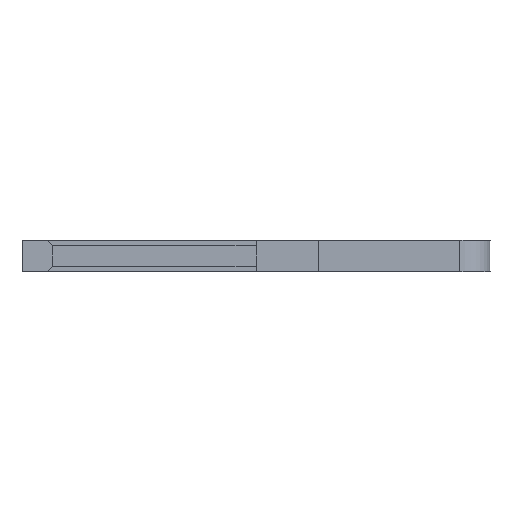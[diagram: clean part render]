
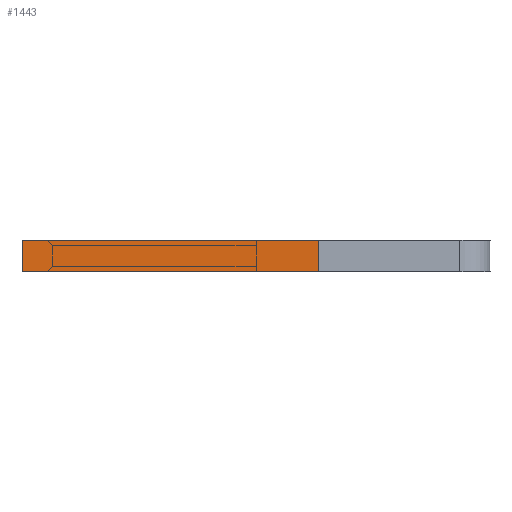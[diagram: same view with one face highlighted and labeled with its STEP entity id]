
A CAD part, left-side view. The second image highlights one B-rep face of the part: STEP entity #1443.
In plain terms, the highlighted face is planar.
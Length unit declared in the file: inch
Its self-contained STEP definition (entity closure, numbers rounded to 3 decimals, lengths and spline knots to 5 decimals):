
#244 = VERTEX_POINT ( 'NONE', #1079 ) ;
#296 = EDGE_CURVE ( 'NONE', #2512, #3378, #2258, .T. ) ;
#384 = DIRECTION ( 'NONE',  ( 0., 1., 0. ) ) ;
#651 = ORIENTED_EDGE ( 'NONE', *, *, #2189, .F. ) ;
#654 = CARTESIAN_POINT ( 'NONE',  ( -0.01, 0.15, -0.04 ) ) ;
#676 = ORIENTED_EDGE ( 'NONE', *, *, #1287, .T. ) ;
#684 = LINE ( 'NONE', #1186, #3525 ) ;
#754 = AXIS2_PLACEMENT_3D ( 'NONE', #3221, #3492, #1765 ) ;
#759 = VECTOR ( 'NONE', #2547, 39.37008 ) ;
#926 = VECTOR ( 'NONE', #384, 39.37008 ) ;
#1079 = CARTESIAN_POINT ( 'NONE',  ( 0.01, 0.15, -0.04 ) ) ;
#1186 = CARTESIAN_POINT ( 'NONE',  ( 0.01, 0.15, -0.04 ) ) ;
#1196 = DIRECTION ( 'NONE',  ( -1., 0., 0. ) ) ;
#1287 = EDGE_CURVE ( 'NONE', #3378, #2867, #2703, .T. ) ;
#1443 = ADVANCED_FACE ( 'NONE', ( #1454 ), #1450, .F. ) ;
#1450 = PLANE ( 'NONE',  #754 ) ;
#1454 = FACE_OUTER_BOUND ( 'NONE', #3390, .T. ) ;
#1765 = DIRECTION ( 'NONE',  ( 1., 0., 0. ) ) ;
#1893 = EDGE_CURVE ( 'NONE', #244, #2867, #684, .T. ) ;
#2053 = ORIENTED_EDGE ( 'NONE', *, *, #1893, .F. ) ;
#2136 = ORIENTED_EDGE ( 'NONE', *, *, #296, .T. ) ;
#2189 = EDGE_CURVE ( 'NONE', #2512, #244, #3687, .T. ) ;
#2258 = LINE ( 'NONE', #3716, #759 ) ;
#2263 = CARTESIAN_POINT ( 'NONE',  ( -0.01, 0.15, -0.04 ) ) ;
#2493 = CARTESIAN_POINT ( 'NONE',  ( -0.01, -0.04, -0.04 ) ) ;
#2512 = VERTEX_POINT ( 'NONE', #3599 ) ;
#2547 = DIRECTION ( 'NONE',  ( -1., 0., 0. ) ) ;
#2554 = DIRECTION ( 'NONE',  ( 0., 1., 0. ) ) ;
#2703 = LINE ( 'NONE', #2263, #3263 ) ;
#2867 = VERTEX_POINT ( 'NONE', #654 ) ;
#3221 = CARTESIAN_POINT ( 'NONE',  ( 0.01, 0.15, -0.04 ) ) ;
#3262 = CARTESIAN_POINT ( 'NONE',  ( 0.01, 0.15, -0.04 ) ) ;
#3263 = VECTOR ( 'NONE', #2554, 39.37008 ) ;
#3378 = VERTEX_POINT ( 'NONE', #2493 ) ;
#3390 = EDGE_LOOP ( 'NONE', ( #676, #2053, #651, #2136 ) ) ;
#3492 = DIRECTION ( 'NONE',  ( 0., 0., 1. ) ) ;
#3525 = VECTOR ( 'NONE', #1196, 39.37008 ) ;
#3599 = CARTESIAN_POINT ( 'NONE',  ( 0.01, -0.04, -0.04 ) ) ;
#3687 = LINE ( 'NONE', #3262, #926 ) ;
#3716 = CARTESIAN_POINT ( 'NONE',  ( 0.01, -0.04, -0.04 ) ) ;
